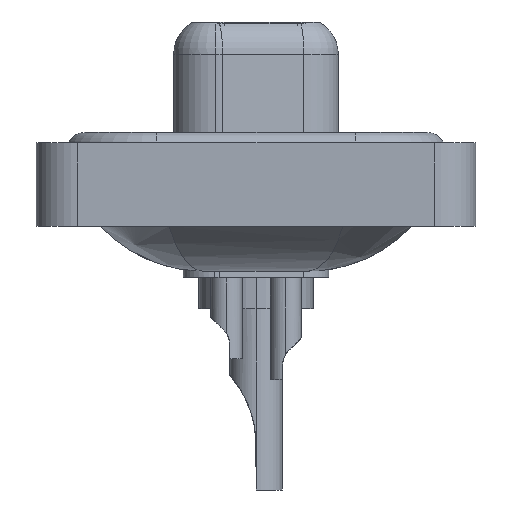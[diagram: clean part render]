
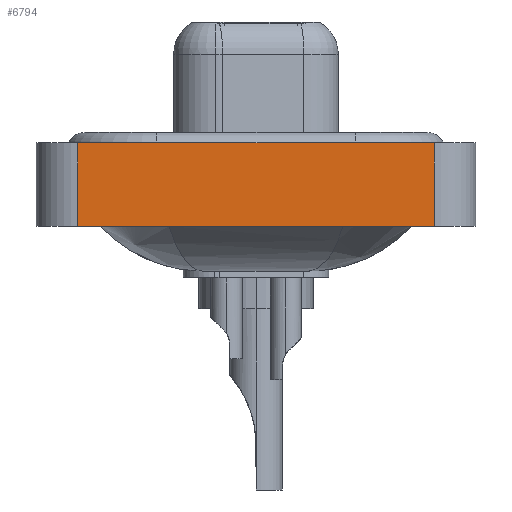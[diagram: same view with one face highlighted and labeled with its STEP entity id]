
A CAD part, left-side view. The second image highlights one B-rep face of the part: STEP entity #6794.
In plain terms, the highlighted planar face has unit normal (-1, 0, 0).
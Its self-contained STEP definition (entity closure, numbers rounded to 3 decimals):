
#305 = AXIS2_PLACEMENT_3D ( 'NONE', #1990, #14108, #9200 ) ;
#398 = EDGE_CURVE ( 'NONE', #17367, #4043, #17513, .T. ) ;
#544 = EDGE_CURVE ( 'NONE', #8605, #14817, #14524, .T. ) ;
#900 = DIRECTION ( 'NONE',  ( 0., 0., 1. ) ) ;
#1714 = CARTESIAN_POINT ( 'NONE',  ( -7.3, -8.55, -3.6 ) ) ;
#1750 = FACE_OUTER_BOUND ( 'NONE', #9599, .T. ) ;
#1990 = CARTESIAN_POINT ( 'NONE',  ( -7.3, -8.55, -3.6 ) ) ;
#2336 = LINE ( 'NONE', #21787, #13704 ) ;
#3849 = ORIENTED_EDGE ( 'NONE', *, *, #13417, .F. ) ;
#4043 = VERTEX_POINT ( 'NONE', #1714 ) ;
#4311 = EDGE_CURVE ( 'NONE', #4043, #14817, #18738, .T. ) ;
#5242 = ORIENTED_EDGE ( 'NONE', *, *, #398, .T. ) ;
#5962 = CARTESIAN_POINT ( 'NONE',  ( -7.3, -8.55, 0.4 ) ) ;
#6794 = ADVANCED_FACE ( 'NONE', ( #1750 ), #21345, .T. ) ;
#7410 = CARTESIAN_POINT ( 'NONE',  ( -7.3, 8.55, 0.4 ) ) ;
#8375 = ORIENTED_EDGE ( 'NONE', *, *, #544, .F. ) ;
#8605 = VERTEX_POINT ( 'NONE', #7410 ) ;
#8934 = CARTESIAN_POINT ( 'NONE',  ( -7.3, -8.55, -3.6 ) ) ;
#9200 = DIRECTION ( 'NONE',  ( 0., 0., 1. ) ) ;
#9322 = DIRECTION ( 'NONE',  ( 0., 0., 1. ) ) ;
#9599 = EDGE_LOOP ( 'NONE', ( #12794, #8375, #3849, #5242 ) ) ;
#9630 = CARTESIAN_POINT ( 'NONE',  ( -7.3, 8.55, -3.6 ) ) ;
#9716 = CARTESIAN_POINT ( 'NONE',  ( -7.3, -8.55, -3.6 ) ) ;
#10709 = VECTOR ( 'NONE', #11191, 1000. ) ;
#11191 = DIRECTION ( 'NONE',  ( 0., -1., 0. ) ) ;
#12794 = ORIENTED_EDGE ( 'NONE', *, *, #4311, .T. ) ;
#13417 = EDGE_CURVE ( 'NONE', #17367, #8605, #2336, .T. ) ;
#13704 = VECTOR ( 'NONE', #9322, 1000. ) ;
#14108 = DIRECTION ( 'NONE',  ( -1., 0., 0. ) ) ;
#14524 = LINE ( 'NONE', #5962, #10709 ) ;
#14817 = VERTEX_POINT ( 'NONE', #22187 ) ;
#15472 = VECTOR ( 'NONE', #16143, 1000. ) ;
#16143 = DIRECTION ( 'NONE',  ( 0., -1., 0. ) ) ;
#17367 = VERTEX_POINT ( 'NONE', #9630 ) ;
#17513 = LINE ( 'NONE', #8934, #15472 ) ;
#18738 = LINE ( 'NONE', #9716, #19479 ) ;
#19479 = VECTOR ( 'NONE', #900, 1000. ) ;
#21345 = PLANE ( 'NONE',  #305 ) ;
#21787 = CARTESIAN_POINT ( 'NONE',  ( -7.3, 8.55, -3.6 ) ) ;
#22187 = CARTESIAN_POINT ( 'NONE',  ( -7.3, -8.55, 0.4 ) ) ;
